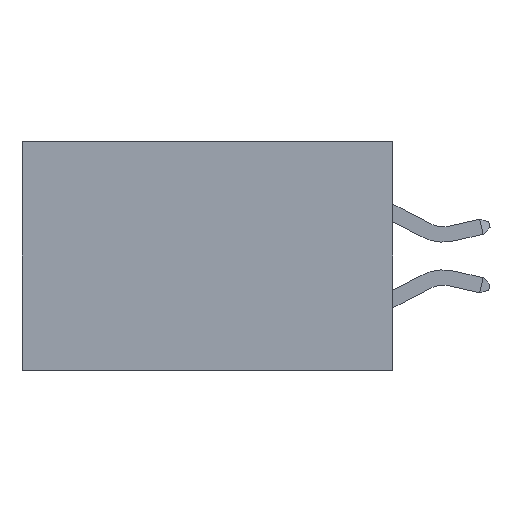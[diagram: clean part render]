
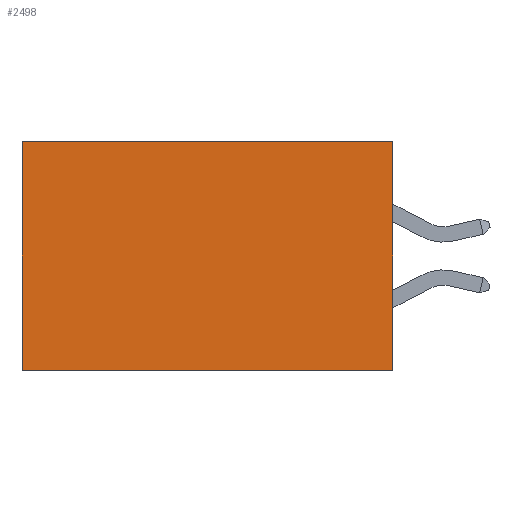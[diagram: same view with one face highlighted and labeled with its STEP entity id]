
A CAD part, left-side view. The second image highlights one B-rep face of the part: STEP entity #2498.
In plain terms, the highlighted planar face has unit normal (-1, 0, 0).
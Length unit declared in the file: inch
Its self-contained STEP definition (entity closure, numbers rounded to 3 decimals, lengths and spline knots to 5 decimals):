
#697 = CARTESIAN_POINT ( 'NONE',  ( 0.2875, 0., 0. ) ) ;
#714 = CARTESIAN_POINT ( 'NONE',  ( 0.2875, 0., -0.37 ) ) ;
#810 = ORIENTED_EDGE ( 'NONE', *, *, #11067, .T. ) ;
#1206 = DIRECTION ( 'NONE',  ( 0., 0., -1. ) ) ;
#1460 = ORIENTED_EDGE ( 'NONE', *, *, #8535, .T. ) ;
#1533 = EDGE_LOOP ( 'NONE', ( #810, #3756, #6504, #1460 ) ) ;
#2339 = LINE ( 'NONE', #697, #13038 ) ;
#2498 = ADVANCED_FACE ( 'NONE', ( #6511 ), #11474, .F. ) ;
#3398 = EDGE_CURVE ( 'NONE', #9898, #8204, #8600, .T. ) ;
#3756 = ORIENTED_EDGE ( 'NONE', *, *, #3398, .F. ) ;
#3999 = CARTESIAN_POINT ( 'NONE',  ( 0.2875, 0., 0. ) ) ;
#4057 = LINE ( 'NONE', #4637, #7160 ) ;
#4158 = EDGE_CURVE ( 'NONE', #10186, #9898, #5315, .T. ) ;
#4637 = CARTESIAN_POINT ( 'NONE',  ( 0.2875, 0.6, 0. ) ) ;
#5315 = LINE ( 'NONE', #9915, #7447 ) ;
#5419 = CARTESIAN_POINT ( 'NONE',  ( 0.2875, 0., 0. ) ) ;
#6504 = ORIENTED_EDGE ( 'NONE', *, *, #4158, .F. ) ;
#6511 = FACE_OUTER_BOUND ( 'NONE', #1533, .T. ) ;
#7160 = VECTOR ( 'NONE', #12831, 39.37008 ) ;
#7399 = AXIS2_PLACEMENT_3D ( 'NONE', #3999, #11372, #11717 ) ;
#7447 = VECTOR ( 'NONE', #1206, 39.37008 ) ;
#8204 = VERTEX_POINT ( 'NONE', #11966 ) ;
#8436 = CARTESIAN_POINT ( 'NONE',  ( 0.2875, 0., -0.37 ) ) ;
#8535 = EDGE_CURVE ( 'NONE', #10186, #12552, #2339, .T. ) ;
#8600 = LINE ( 'NONE', #8436, #10994 ) ;
#8750 = DIRECTION ( 'NONE',  ( 0., 1., 0. ) ) ;
#9636 = CARTESIAN_POINT ( 'NONE',  ( 0.2875, 0.6, 0. ) ) ;
#9898 = VERTEX_POINT ( 'NONE', #714 ) ;
#9915 = CARTESIAN_POINT ( 'NONE',  ( 0.2875, 0., 0. ) ) ;
#10186 = VERTEX_POINT ( 'NONE', #5419 ) ;
#10199 = DIRECTION ( 'NONE',  ( 0., 1., 0. ) ) ;
#10994 = VECTOR ( 'NONE', #8750, 39.37008 ) ;
#11067 = EDGE_CURVE ( 'NONE', #12552, #8204, #4057, .T. ) ;
#11372 = DIRECTION ( 'NONE',  ( 1., 0., 0. ) ) ;
#11474 = PLANE ( 'NONE',  #7399 ) ;
#11717 = DIRECTION ( 'NONE',  ( 0., 0., -1. ) ) ;
#11966 = CARTESIAN_POINT ( 'NONE',  ( 0.2875, 0.6, -0.37 ) ) ;
#12552 = VERTEX_POINT ( 'NONE', #9636 ) ;
#12831 = DIRECTION ( 'NONE',  ( 0., 0., -1. ) ) ;
#13038 = VECTOR ( 'NONE', #10199, 39.37008 ) ;
